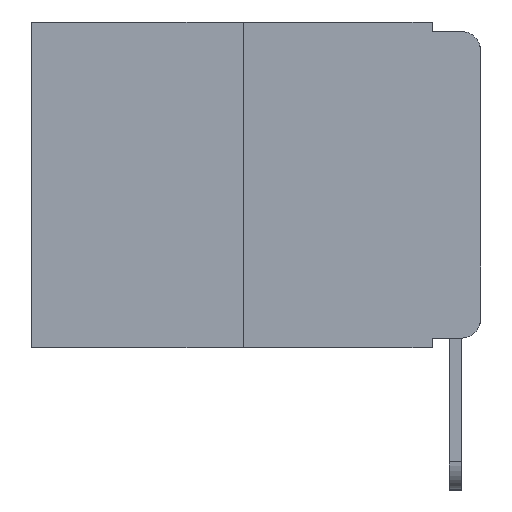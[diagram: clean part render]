
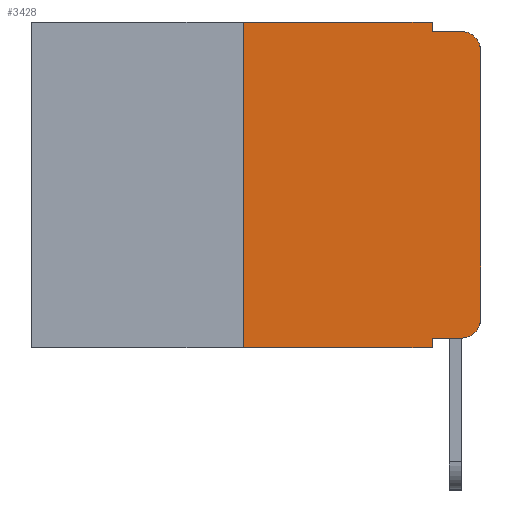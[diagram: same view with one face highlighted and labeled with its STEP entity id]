
A CAD part, left-side view. The second image highlights one B-rep face of the part: STEP entity #3428.
In plain terms, the highlighted planar face has unit normal (-1, 0, 0).
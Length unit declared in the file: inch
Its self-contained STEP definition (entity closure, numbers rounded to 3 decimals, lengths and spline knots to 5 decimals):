
#410 = VERTEX_POINT ( 'NONE', #19903 ) ;
#465 = CARTESIAN_POINT ( 'NONE',  ( 0., 0.051, -0.333 ) ) ;
#1067 = ORIENTED_EDGE ( 'NONE', *, *, #10092, .F. ) ;
#1223 = DIRECTION ( 'NONE',  ( -1., 0., 0. ) ) ;
#1255 = CIRCLE ( 'NONE', #7480, 0.02 ) ;
#1366 = CARTESIAN_POINT ( 'NONE',  ( 0., 0.051, 0. ) ) ;
#2444 = DIRECTION ( 'NONE',  ( 0., -1., 0. ) ) ;
#3129 = DIRECTION ( 'NONE',  ( 0., -1., 0. ) ) ;
#3262 = ORIENTED_EDGE ( 'NONE', *, *, #15566, .T. ) ;
#3428 = ADVANCED_FACE ( 'NONE', ( #4635 ), #14981, .F. ) ;
#3508 = LINE ( 'NONE', #1366, #16587 ) ;
#3586 = EDGE_LOOP ( 'NONE', ( #20171, #3262, #12528, #9250, #5035, #1067, #10784, #6850, #11304, #20438 ) ) ;
#3704 = LINE ( 'NONE', #465, #21061 ) ;
#4235 = LINE ( 'NONE', #19668, #12851 ) ;
#4249 = CARTESIAN_POINT ( 'NONE',  ( 0., 0.02, -0.01 ) ) ;
#4635 = FACE_OUTER_BOUND ( 'NONE', #3586, .T. ) ;
#5035 = ORIENTED_EDGE ( 'NONE', *, *, #18993, .F. ) ;
#5293 = DIRECTION ( 'NONE',  ( 0., 0., -1. ) ) ;
#5531 = CARTESIAN_POINT ( 'NONE',  ( 0., 0.051, -0.01 ) ) ;
#6479 = VERTEX_POINT ( 'NONE', #4249 ) ;
#6685 = EDGE_CURVE ( 'NONE', #11915, #12928, #1255, .T. ) ;
#6761 = DIRECTION ( 'NONE',  ( 0., 0., -1. ) ) ;
#6850 = ORIENTED_EDGE ( 'NONE', *, *, #8996, .F. ) ;
#6923 = DIRECTION ( 'NONE',  ( 0., 0., -1. ) ) ;
#7150 = VECTOR ( 'NONE', #3129, 39.37008 ) ;
#7480 = AXIS2_PLACEMENT_3D ( 'NONE', #18710, #8934, #20299 ) ;
#7794 = VECTOR ( 'NONE', #13406, 39.37008 ) ;
#7863 = EDGE_CURVE ( 'NONE', #21241, #11915, #3704, .T. ) ;
#8610 = CARTESIAN_POINT ( 'NONE',  ( 0., 0.473, -0.343 ) ) ;
#8934 = DIRECTION ( 'NONE',  ( -1., 0., 0. ) ) ;
#8996 = EDGE_CURVE ( 'NONE', #21241, #410, #3508, .T. ) ;
#9166 = VECTOR ( 'NONE', #6923, 39.37008 ) ;
#9206 = DIRECTION ( 'NONE',  ( 0., 0., 1. ) ) ;
#9250 = ORIENTED_EDGE ( 'NONE', *, *, #12256, .F. ) ;
#9703 = LINE ( 'NONE', #10321, #9166 ) ;
#10092 = EDGE_CURVE ( 'NONE', #20136, #22180, #20572, .T. ) ;
#10321 = CARTESIAN_POINT ( 'NONE',  ( 0., 0.051, 0. ) ) ;
#10661 = AXIS2_PLACEMENT_3D ( 'NONE', #19797, #16628, #6761 ) ;
#10784 = ORIENTED_EDGE ( 'NONE', *, *, #21245, .T. ) ;
#11304 = ORIENTED_EDGE ( 'NONE', *, *, #7863, .T. ) ;
#11646 = CARTESIAN_POINT ( 'NONE',  ( 0., 0.25, -0.343 ) ) ;
#11915 = VERTEX_POINT ( 'NONE', #14570 ) ;
#12002 = CARTESIAN_POINT ( 'NONE',  ( 0., 0.02, -0.03 ) ) ;
#12086 = LINE ( 'NONE', #8610, #7150 ) ;
#12163 = LINE ( 'NONE', #19911, #7794 ) ;
#12256 = EDGE_CURVE ( 'NONE', #12972, #18479, #9703, .T. ) ;
#12528 = ORIENTED_EDGE ( 'NONE', *, *, #14413, .F. ) ;
#12851 = VECTOR ( 'NONE', #18076, 39.37008 ) ;
#12928 = VERTEX_POINT ( 'NONE', #19664 ) ;
#12972 = VERTEX_POINT ( 'NONE', #13231 ) ;
#13206 = CIRCLE ( 'NONE', #16382, 0.02 ) ;
#13231 = CARTESIAN_POINT ( 'NONE',  ( 0., 0.051, 0. ) ) ;
#13380 = LINE ( 'NONE', #19222, #13891 ) ;
#13406 = DIRECTION ( 'NONE',  ( 0., -1., 0. ) ) ;
#13418 = CARTESIAN_POINT ( 'NONE',  ( 0., 0.051, -0.333 ) ) ;
#13580 = DIRECTION ( 'NONE',  ( 0., 0., -1. ) ) ;
#13891 = VECTOR ( 'NONE', #20836, 39.37008 ) ;
#14413 = EDGE_CURVE ( 'NONE', #18479, #6479, #12163, .T. ) ;
#14570 = CARTESIAN_POINT ( 'NONE',  ( 0., 0.02, -0.333 ) ) ;
#14919 = CARTESIAN_POINT ( 'NONE',  ( 0., 0.25, 0. ) ) ;
#14981 = PLANE ( 'NONE',  #10661 ) ;
#15566 = EDGE_CURVE ( 'NONE', #18605, #6479, #13206, .T. ) ;
#15688 = CARTESIAN_POINT ( 'NONE',  ( 0., 0.25, 0. ) ) ;
#16280 = VECTOR ( 'NONE', #9206, 39.37008 ) ;
#16382 = AXIS2_PLACEMENT_3D ( 'NONE', #12002, #1223, #13580 ) ;
#16587 = VECTOR ( 'NONE', #5293, 39.37008 ) ;
#16628 = DIRECTION ( 'NONE',  ( 1., 0., 0. ) ) ;
#17733 = EDGE_CURVE ( 'NONE', #12928, #18605, #13380, .T. ) ;
#18076 = DIRECTION ( 'NONE',  ( 0., -1., 0. ) ) ;
#18479 = VERTEX_POINT ( 'NONE', #5531 ) ;
#18605 = VERTEX_POINT ( 'NONE', #22259 ) ;
#18710 = CARTESIAN_POINT ( 'NONE',  ( 0., 0.02, -0.313 ) ) ;
#18993 = EDGE_CURVE ( 'NONE', #22180, #12972, #4235, .T. ) ;
#19222 = CARTESIAN_POINT ( 'NONE',  ( 0., 0., 0. ) ) ;
#19664 = CARTESIAN_POINT ( 'NONE',  ( 0., 0., -0.313 ) ) ;
#19668 = CARTESIAN_POINT ( 'NONE',  ( 0., 0.473, 0. ) ) ;
#19797 = CARTESIAN_POINT ( 'NONE',  ( 0., 0.473, 0. ) ) ;
#19903 = CARTESIAN_POINT ( 'NONE',  ( 0., 0.051, -0.343 ) ) ;
#19911 = CARTESIAN_POINT ( 'NONE',  ( 0., 0.051, -0.01 ) ) ;
#20136 = VERTEX_POINT ( 'NONE', #11646 ) ;
#20171 = ORIENTED_EDGE ( 'NONE', *, *, #17733, .T. ) ;
#20299 = DIRECTION ( 'NONE',  ( 0., 0., -1. ) ) ;
#20438 = ORIENTED_EDGE ( 'NONE', *, *, #6685, .T. ) ;
#20572 = LINE ( 'NONE', #15688, #16280 ) ;
#20836 = DIRECTION ( 'NONE',  ( 0., 0., 1. ) ) ;
#21061 = VECTOR ( 'NONE', #2444, 39.37008 ) ;
#21241 = VERTEX_POINT ( 'NONE', #13418 ) ;
#21245 = EDGE_CURVE ( 'NONE', #20136, #410, #12086, .T. ) ;
#22180 = VERTEX_POINT ( 'NONE', #14919 ) ;
#22259 = CARTESIAN_POINT ( 'NONE',  ( 0., 0., -0.03 ) ) ;
